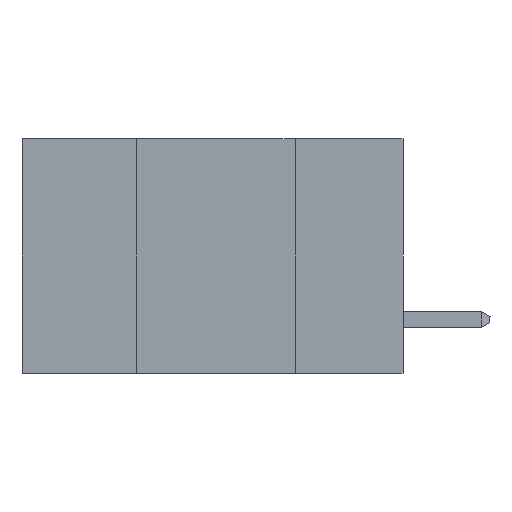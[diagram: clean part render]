
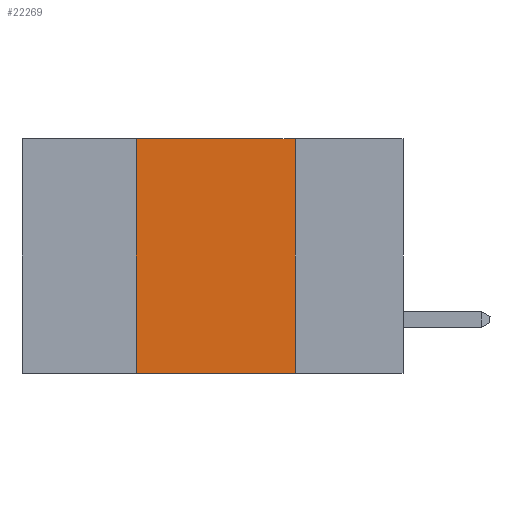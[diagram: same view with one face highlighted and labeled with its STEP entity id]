
A CAD part, left-side view. The second image highlights one B-rep face of the part: STEP entity #22269.
In plain terms, the highlighted planar face has unit normal (-1, 0, 0).
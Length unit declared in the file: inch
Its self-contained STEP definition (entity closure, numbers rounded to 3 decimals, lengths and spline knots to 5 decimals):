
#2008 = FACE_OUTER_BOUND ( 'NONE', #20545, .T. ) ;
#2450 = ORIENTED_EDGE ( 'NONE', *, *, #26427, .F. ) ;
#2535 = ORIENTED_EDGE ( 'NONE', *, *, #11156, .T. ) ;
#3677 = DIRECTION ( 'NONE',  ( 0., -1., 0. ) ) ;
#3807 = DIRECTION ( 'NONE',  ( 0., 0., -1. ) ) ;
#4435 = DIRECTION ( 'NONE',  ( 0., -1., 0. ) ) ;
#5213 = VECTOR ( 'NONE', #3677, 39.37008 ) ;
#5732 = CARTESIAN_POINT ( 'NONE',  ( 0., 0.42, 0. ) ) ;
#5938 = EDGE_CURVE ( 'NONE', #25228, #15259, #27469, .T. ) ;
#7457 = AXIS2_PLACEMENT_3D ( 'NONE', #23415, #16372, #21502 ) ;
#10968 = CARTESIAN_POINT ( 'NONE',  ( 0., 0.42, -0.37 ) ) ;
#11156 = EDGE_CURVE ( 'NONE', #25228, #16908, #14167, .T. ) ;
#11743 = PLANE ( 'NONE',  #7457 ) ;
#14167 = LINE ( 'NONE', #18494, #22365 ) ;
#15259 = VERTEX_POINT ( 'NONE', #18722 ) ;
#15512 = ORIENTED_EDGE ( 'NONE', *, *, #15590, .F. ) ;
#15590 = EDGE_CURVE ( 'NONE', #15259, #29998, #27959, .T. ) ;
#16241 = VECTOR ( 'NONE', #3807, 39.37008 ) ;
#16372 = DIRECTION ( 'NONE',  ( 1., 0., 0. ) ) ;
#16908 = VERTEX_POINT ( 'NONE', #23326 ) ;
#17230 = ORIENTED_EDGE ( 'NONE', *, *, #5938, .F. ) ;
#18494 = CARTESIAN_POINT ( 'NONE',  ( 0., 0.6, -0.37 ) ) ;
#18722 = CARTESIAN_POINT ( 'NONE',  ( 0., 0.42, 0. ) ) ;
#20274 = DIRECTION ( 'NONE',  ( 0., 0., 1. ) ) ;
#20545 = EDGE_LOOP ( 'NONE', ( #2450, #15512, #17230, #2535 ) ) ;
#21502 = DIRECTION ( 'NONE',  ( 0., 0., -1. ) ) ;
#22269 = ADVANCED_FACE ( 'NONE', ( #2008 ), #11743, .F. ) ;
#22365 = VECTOR ( 'NONE', #4435, 39.37008 ) ;
#23326 = CARTESIAN_POINT ( 'NONE',  ( 0., 0.17, -0.37 ) ) ;
#23415 = CARTESIAN_POINT ( 'NONE',  ( 0., 0.6, 0. ) ) ;
#23606 = LINE ( 'NONE', #28405, #16241 ) ;
#25228 = VERTEX_POINT ( 'NONE', #10968 ) ;
#25558 = CARTESIAN_POINT ( 'NONE',  ( 0., 0.6, 0. ) ) ;
#26427 = EDGE_CURVE ( 'NONE', #29998, #16908, #23606, .T. ) ;
#27469 = LINE ( 'NONE', #5732, #30226 ) ;
#27959 = LINE ( 'NONE', #25558, #5213 ) ;
#28405 = CARTESIAN_POINT ( 'NONE',  ( 0., 0.17, 0. ) ) ;
#29217 = CARTESIAN_POINT ( 'NONE',  ( 0., 0.17, 0. ) ) ;
#29998 = VERTEX_POINT ( 'NONE', #29217 ) ;
#30226 = VECTOR ( 'NONE', #20274, 39.37008 ) ;
